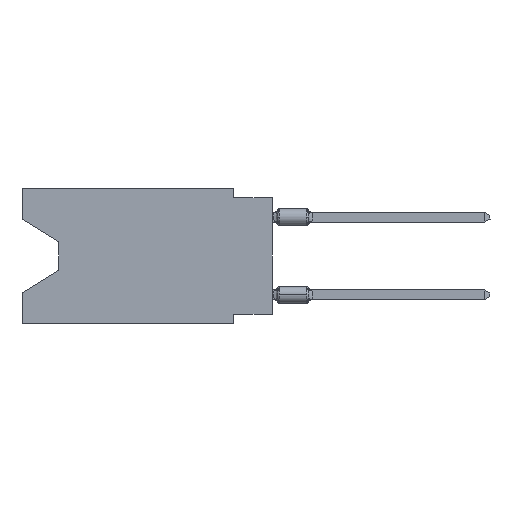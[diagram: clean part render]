
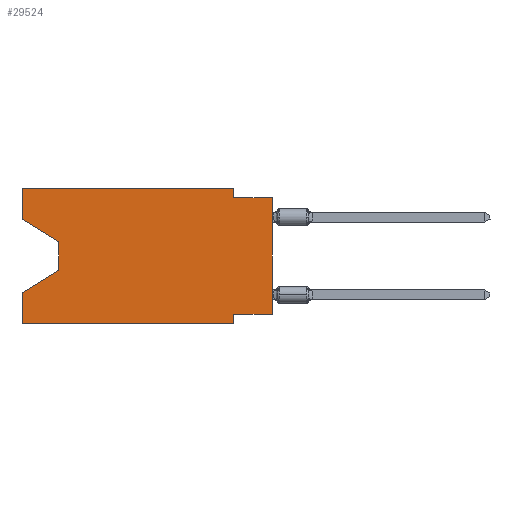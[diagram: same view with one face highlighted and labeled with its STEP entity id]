
A CAD part, left-side view. The second image highlights one B-rep face of the part: STEP entity #29524.
In plain terms, the highlighted planar face has unit normal (-1, 0, 0).
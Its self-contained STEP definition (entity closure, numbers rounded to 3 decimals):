
#389 = DIRECTION ( 'NONE',  ( 0., 0.855, -0.519 ) ) ;
#536 = CARTESIAN_POINT ( 'NONE',  ( 0., 16.383, 0. ) ) ;
#1161 = CARTESIAN_POINT ( 'NONE',  ( 0., 16.383, 0. ) ) ;
#1263 = LINE ( 'NONE', #23905, #33194 ) ;
#1487 = DIRECTION ( 'NONE',  ( 0., -0.855, -0.519 ) ) ;
#1880 = VERTEX_POINT ( 'NONE', #2775 ) ;
#2319 = EDGE_CURVE ( 'NONE', #16528, #14800, #19265, .T. ) ;
#2775 = CARTESIAN_POINT ( 'NONE',  ( 0., 0., -0.635 ) ) ;
#3095 = CARTESIAN_POINT ( 'NONE',  ( 0., 2.54, 0. ) ) ;
#3283 = CARTESIAN_POINT ( 'NONE',  ( 0., 13.97, -5.385 ) ) ;
#3570 = ORIENTED_EDGE ( 'NONE', *, *, #31574, .F. ) ;
#3664 = ORIENTED_EDGE ( 'NONE', *, *, #28730, .F. ) ;
#3796 = CARTESIAN_POINT ( 'NONE',  ( 0., 13.97, -3.505 ) ) ;
#4682 = DIRECTION ( 'NONE',  ( 0., -1., 0. ) ) ;
#4821 = EDGE_CURVE ( 'NONE', #19039, #19852, #18055, .T. ) ;
#5147 = ORIENTED_EDGE ( 'NONE', *, *, #11722, .T. ) ;
#5414 = CARTESIAN_POINT ( 'NONE',  ( 0., 0., -0.635 ) ) ;
#5727 = CARTESIAN_POINT ( 'NONE',  ( 0., 0., -8.255 ) ) ;
#6650 = DIRECTION ( 'NONE',  ( 0., 0., 1. ) ) ;
#7674 = LINE ( 'NONE', #36096, #36571 ) ;
#7749 = VERTEX_POINT ( 'NONE', #3095 ) ;
#7826 = ORIENTED_EDGE ( 'NONE', *, *, #36366, .F. ) ;
#7859 = CARTESIAN_POINT ( 'NONE',  ( 0., 16.383, -8.89 ) ) ;
#8477 = CARTESIAN_POINT ( 'NONE',  ( 0., 2.54, -8.89 ) ) ;
#9253 = CARTESIAN_POINT ( 'NONE',  ( 0., 0., 0. ) ) ;
#9429 = VECTOR ( 'NONE', #25513, 1000. ) ;
#9612 = LINE ( 'NONE', #9253, #24702 ) ;
#9631 = ORIENTED_EDGE ( 'NONE', *, *, #21966, .T. ) ;
#9931 = VERTEX_POINT ( 'NONE', #20548 ) ;
#10009 = FACE_OUTER_BOUND ( 'NONE', #16197, .T. ) ;
#10473 = DIRECTION ( 'NONE',  ( 0., -1., 0. ) ) ;
#10668 = VERTEX_POINT ( 'NONE', #3796 ) ;
#11722 = EDGE_CURVE ( 'NONE', #20675, #14800, #28283, .T. ) ;
#14057 = DIRECTION ( 'NONE',  ( 0., 0., -1. ) ) ;
#14193 = CARTESIAN_POINT ( 'NONE',  ( 0., 16.383, -8.89 ) ) ;
#14700 = VECTOR ( 'NONE', #14057, 1000. ) ;
#14800 = VERTEX_POINT ( 'NONE', #18681 ) ;
#15371 = CARTESIAN_POINT ( 'NONE',  ( 0., 2.54, -0.635 ) ) ;
#15799 = EDGE_CURVE ( 'NONE', #20675, #9931, #1263, .T. ) ;
#15875 = LINE ( 'NONE', #18477, #28589 ) ;
#16197 = EDGE_LOOP ( 'NONE', ( #9631, #16889, #27821, #18570, #5147, #19305, #7826, #21488, #17309, #3664, #3570, #34934 ) ) ;
#16215 = DIRECTION ( 'NONE',  ( 0., 0., -1. ) ) ;
#16528 = VERTEX_POINT ( 'NONE', #19383 ) ;
#16889 = ORIENTED_EDGE ( 'NONE', *, *, #31346, .T. ) ;
#16978 = VERTEX_POINT ( 'NONE', #15371 ) ;
#17200 = LINE ( 'NONE', #22755, #32094 ) ;
#17309 = ORIENTED_EDGE ( 'NONE', *, *, #30289, .F. ) ;
#18055 = LINE ( 'NONE', #1161, #30207 ) ;
#18477 = CARTESIAN_POINT ( 'NONE',  ( 0., 16.383, 0. ) ) ;
#18570 = ORIENTED_EDGE ( 'NONE', *, *, #15799, .F. ) ;
#18681 = CARTESIAN_POINT ( 'NONE',  ( 0., 2.54, -8.89 ) ) ;
#19039 = VERTEX_POINT ( 'NONE', #30713 ) ;
#19265 = LINE ( 'NONE', #8477, #14700 ) ;
#19281 = CARTESIAN_POINT ( 'NONE',  ( 0., 16.383, 0. ) ) ;
#19305 = ORIENTED_EDGE ( 'NONE', *, *, #2319, .F. ) ;
#19383 = CARTESIAN_POINT ( 'NONE',  ( 0., 2.54, -8.255 ) ) ;
#19852 = VERTEX_POINT ( 'NONE', #536 ) ;
#19987 = DIRECTION ( 'NONE',  ( 0., 0., -1. ) ) ;
#20548 = CARTESIAN_POINT ( 'NONE',  ( 0., 16.383, -6.852 ) ) ;
#20675 = VERTEX_POINT ( 'NONE', #7859 ) ;
#20921 = VECTOR ( 'NONE', #19987, 1000. ) ;
#21488 = ORIENTED_EDGE ( 'NONE', *, *, #30930, .T. ) ;
#21731 = AXIS2_PLACEMENT_3D ( 'NONE', #19281, #30583, #35641 ) ;
#21966 = EDGE_CURVE ( 'NONE', #19039, #10668, #29679, .T. ) ;
#22390 = CARTESIAN_POINT ( 'NONE',  ( 0., 13.97, -3.505 ) ) ;
#22755 = CARTESIAN_POINT ( 'NONE',  ( 0., 0., -8.255 ) ) ;
#23361 = DIRECTION ( 'NONE',  ( 0., 0., 1. ) ) ;
#23580 = VECTOR ( 'NONE', #4682, 1000. ) ;
#23905 = CARTESIAN_POINT ( 'NONE',  ( 0., 16.383, 0. ) ) ;
#24416 = EDGE_CURVE ( 'NONE', #32540, #9931, #31556, .T. ) ;
#24702 = VECTOR ( 'NONE', #23361, 1000. ) ;
#25513 = DIRECTION ( 'NONE',  ( 0., -1., 0. ) ) ;
#26903 = CARTESIAN_POINT ( 'NONE',  ( 0., 16.383, -2.038 ) ) ;
#27821 = ORIENTED_EDGE ( 'NONE', *, *, #24416, .T. ) ;
#28217 = VECTOR ( 'NONE', #1487, 1000. ) ;
#28283 = LINE ( 'NONE', #14193, #9429 ) ;
#28589 = VECTOR ( 'NONE', #10473, 1000. ) ;
#28730 = EDGE_CURVE ( 'NONE', #7749, #16978, #7674, .T. ) ;
#29282 = VECTOR ( 'NONE', #389, 1000. ) ;
#29524 = ADVANCED_FACE ( 'NONE', ( #10009 ), #30033, .F. ) ;
#29679 = LINE ( 'NONE', #26903, #28217 ) ;
#30033 = PLANE ( 'NONE',  #21731 ) ;
#30207 = VECTOR ( 'NONE', #35136, 1000. ) ;
#30289 = EDGE_CURVE ( 'NONE', #16978, #1880, #30818, .T. ) ;
#30583 = DIRECTION ( 'NONE',  ( 1., 0., 0. ) ) ;
#30713 = CARTESIAN_POINT ( 'NONE',  ( 0., 16.383, -2.038 ) ) ;
#30818 = LINE ( 'NONE', #5414, #23580 ) ;
#30930 = EDGE_CURVE ( 'NONE', #35798, #1880, #9612, .T. ) ;
#31346 = EDGE_CURVE ( 'NONE', #10668, #32540, #34081, .T. ) ;
#31367 = CARTESIAN_POINT ( 'NONE',  ( 0., 13.97, -5.385 ) ) ;
#31556 = LINE ( 'NONE', #31367, #29282 ) ;
#31574 = EDGE_CURVE ( 'NONE', #19852, #7749, #15875, .T. ) ;
#32094 = VECTOR ( 'NONE', #34078, 1000. ) ;
#32540 = VERTEX_POINT ( 'NONE', #3283 ) ;
#33194 = VECTOR ( 'NONE', #6650, 1000. ) ;
#34078 = DIRECTION ( 'NONE',  ( 0., 1., 0. ) ) ;
#34081 = LINE ( 'NONE', #22390, #20921 ) ;
#34934 = ORIENTED_EDGE ( 'NONE', *, *, #4821, .F. ) ;
#35136 = DIRECTION ( 'NONE',  ( 0., 0., 1. ) ) ;
#35641 = DIRECTION ( 'NONE',  ( 0., 0., -1. ) ) ;
#35798 = VERTEX_POINT ( 'NONE', #5727 ) ;
#36096 = CARTESIAN_POINT ( 'NONE',  ( 0., 2.54, 0. ) ) ;
#36366 = EDGE_CURVE ( 'NONE', #35798, #16528, #17200, .T. ) ;
#36571 = VECTOR ( 'NONE', #16215, 1000. ) ;
